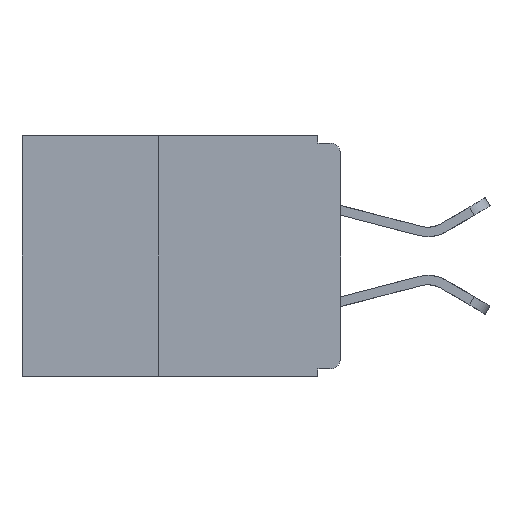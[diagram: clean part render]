
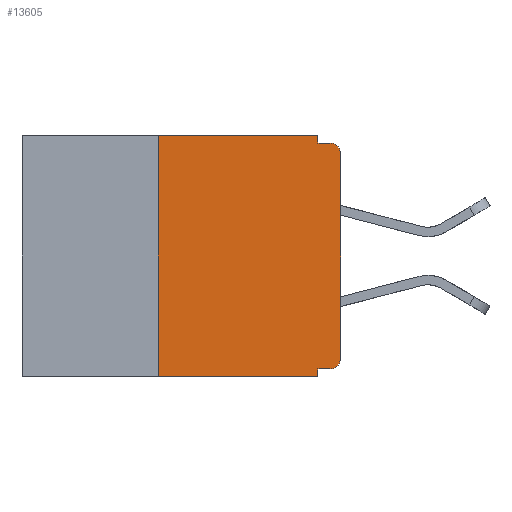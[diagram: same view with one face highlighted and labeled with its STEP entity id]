
A CAD part, left-side view. The second image highlights one B-rep face of the part: STEP entity #13605.
In plain terms, the highlighted planar face has unit normal (-1, 0, 0).
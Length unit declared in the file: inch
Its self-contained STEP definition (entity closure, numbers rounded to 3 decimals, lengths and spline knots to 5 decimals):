
#101 = EDGE_CURVE ( 'NONE', #22698, #2050, #8206, .T. ) ;
#167 = VECTOR ( 'NONE', #7514, 39.37008 ) ;
#479 = VERTEX_POINT ( 'NONE', #2441 ) ;
#530 = CARTESIAN_POINT ( 'NONE',  ( 0., 0., 0. ) ) ;
#1321 = CARTESIAN_POINT ( 'NONE',  ( 0., 0., -0.32 ) ) ;
#1730 = DIRECTION ( 'NONE',  ( 0., 0., -1. ) ) ;
#1799 = CARTESIAN_POINT ( 'NONE',  ( 0., 0.015, -0.025 ) ) ;
#2050 = VERTEX_POINT ( 'NONE', #16902 ) ;
#2095 = AXIS2_PLACEMENT_3D ( 'NONE', #2664, #7198, #19020 ) ;
#2288 = CARTESIAN_POINT ( 'NONE',  ( 0., 0.031, -0.32 ) ) ;
#2322 = LINE ( 'NONE', #14451, #21043 ) ;
#2324 = CARTESIAN_POINT ( 'NONE',  ( 0., 0.031, 0. ) ) ;
#2441 = CARTESIAN_POINT ( 'NONE',  ( 0., 0.015, -0.01 ) ) ;
#2648 = VERTEX_POINT ( 'NONE', #6542 ) ;
#2664 = CARTESIAN_POINT ( 'NONE',  ( 0., 0.015, -0.305 ) ) ;
#3255 = CARTESIAN_POINT ( 'NONE',  ( 0., 0.015, -0.32 ) ) ;
#3269 = DIRECTION ( 'NONE',  ( 0., 0., 1. ) ) ;
#3593 = ORIENTED_EDGE ( 'NONE', *, *, #8871, .F. ) ;
#3656 = DIRECTION ( 'NONE',  ( 0., 0., -1. ) ) ;
#3902 = EDGE_CURVE ( 'NONE', #22698, #8123, #21033, .T. ) ;
#4075 = VERTEX_POINT ( 'NONE', #5519 ) ;
#4183 = ORIENTED_EDGE ( 'NONE', *, *, #18935, .F. ) ;
#4959 = DIRECTION ( 'NONE',  ( 0., -1., 0. ) ) ;
#5228 = LINE ( 'NONE', #10748, #9482 ) ;
#5302 = LINE ( 'NONE', #22932, #19164 ) ;
#5373 = EDGE_CURVE ( 'NONE', #8123, #13644, #2322, .T. ) ;
#5519 = CARTESIAN_POINT ( 'NONE',  ( 0., 0.031, -0.01 ) ) ;
#5787 = EDGE_CURVE ( 'NONE', #16566, #9627, #17944, .T. ) ;
#6329 = EDGE_CURVE ( 'NONE', #2050, #7397, #15070, .T. ) ;
#6542 = CARTESIAN_POINT ( 'NONE',  ( 0., 0.031, 0. ) ) ;
#6786 = DIRECTION ( 'NONE',  ( 0., 1., 0. ) ) ;
#7198 = DIRECTION ( 'NONE',  ( -1., 0., 0. ) ) ;
#7209 = VECTOR ( 'NONE', #6786, 39.37008 ) ;
#7397 = VERTEX_POINT ( 'NONE', #16318 ) ;
#7514 = DIRECTION ( 'NONE',  ( 0., -1., 0. ) ) ;
#7894 = DIRECTION ( 'NONE',  ( 0., 0., 1. ) ) ;
#8123 = VERTEX_POINT ( 'NONE', #2288 ) ;
#8206 = CIRCLE ( 'NONE', #2095, 0.015 ) ;
#8225 = DIRECTION ( 'NONE',  ( 0., 0., -1. ) ) ;
#8871 = EDGE_CURVE ( 'NONE', #4075, #479, #18907, .T. ) ;
#9482 = VECTOR ( 'NONE', #12556, 39.37008 ) ;
#9627 = VERTEX_POINT ( 'NONE', #9699 ) ;
#9699 = CARTESIAN_POINT ( 'NONE',  ( 0., 0.25, 0. ) ) ;
#10141 = CARTESIAN_POINT ( 'NONE',  ( 0., 0.031, -0.33 ) ) ;
#10281 = VECTOR ( 'NONE', #7894, 39.37008 ) ;
#10460 = ORIENTED_EDGE ( 'NONE', *, *, #3902, .F. ) ;
#10507 = AXIS2_PLACEMENT_3D ( 'NONE', #1799, #14515, #3656 ) ;
#10579 = CARTESIAN_POINT ( 'NONE',  ( 0., 0.25, -0.33 ) ) ;
#10717 = AXIS2_PLACEMENT_3D ( 'NONE', #15425, #19064, #8225 ) ;
#10748 = CARTESIAN_POINT ( 'NONE',  ( 0., 0.437, -0.33 ) ) ;
#11400 = EDGE_LOOP ( 'NONE', ( #13207, #20298, #3593, #4183, #23113, #11551, #11854, #22020, #10460, #12442 ) ) ;
#11551 = ORIENTED_EDGE ( 'NONE', *, *, #5787, .F. ) ;
#11854 = ORIENTED_EDGE ( 'NONE', *, *, #22129, .T. ) ;
#12442 = ORIENTED_EDGE ( 'NONE', *, *, #101, .T. ) ;
#12551 = VECTOR ( 'NONE', #3269, 39.37008 ) ;
#12556 = DIRECTION ( 'NONE',  ( 0., -1., 0. ) ) ;
#12566 = EDGE_CURVE ( 'NONE', #9627, #2648, #5302, .T. ) ;
#13207 = ORIENTED_EDGE ( 'NONE', *, *, #6329, .T. ) ;
#13605 = ADVANCED_FACE ( 'NONE', ( #21943 ), #22583, .F. ) ;
#13644 = VERTEX_POINT ( 'NONE', #10141 ) ;
#14451 = CARTESIAN_POINT ( 'NONE',  ( 0., 0.031, -0.33 ) ) ;
#14515 = DIRECTION ( 'NONE',  ( -1., 0., 0. ) ) ;
#15070 = LINE ( 'NONE', #530, #10281 ) ;
#15425 = CARTESIAN_POINT ( 'NONE',  ( 0., 0.437, 0. ) ) ;
#16077 = CARTESIAN_POINT ( 'NONE',  ( 0., 0.25, -0.33 ) ) ;
#16318 = CARTESIAN_POINT ( 'NONE',  ( 0., 0., -0.025 ) ) ;
#16566 = VERTEX_POINT ( 'NONE', #16077 ) ;
#16868 = DIRECTION ( 'NONE',  ( 0., 0., -1. ) ) ;
#16902 = CARTESIAN_POINT ( 'NONE',  ( 0., 0., -0.305 ) ) ;
#16950 = LINE ( 'NONE', #2324, #22288 ) ;
#17180 = CIRCLE ( 'NONE', #10507, 0.015 ) ;
#17944 = LINE ( 'NONE', #10579, #12551 ) ;
#18907 = LINE ( 'NONE', #21954, #167 ) ;
#18935 = EDGE_CURVE ( 'NONE', #2648, #4075, #16950, .T. ) ;
#19020 = DIRECTION ( 'NONE',  ( 0., 0., -1. ) ) ;
#19064 = DIRECTION ( 'NONE',  ( 1., 0., 0. ) ) ;
#19164 = VECTOR ( 'NONE', #4959, 39.37008 ) ;
#20012 = EDGE_CURVE ( 'NONE', #7397, #479, #17180, .T. ) ;
#20298 = ORIENTED_EDGE ( 'NONE', *, *, #20012, .T. ) ;
#21033 = LINE ( 'NONE', #1321, #7209 ) ;
#21043 = VECTOR ( 'NONE', #1730, 39.37008 ) ;
#21943 = FACE_OUTER_BOUND ( 'NONE', #11400, .T. ) ;
#21954 = CARTESIAN_POINT ( 'NONE',  ( 0., 0., -0.01 ) ) ;
#22020 = ORIENTED_EDGE ( 'NONE', *, *, #5373, .F. ) ;
#22129 = EDGE_CURVE ( 'NONE', #16566, #13644, #5228, .T. ) ;
#22288 = VECTOR ( 'NONE', #16868, 39.37008 ) ;
#22583 = PLANE ( 'NONE',  #10717 ) ;
#22698 = VERTEX_POINT ( 'NONE', #3255 ) ;
#22932 = CARTESIAN_POINT ( 'NONE',  ( 0., 0.437, 0. ) ) ;
#23113 = ORIENTED_EDGE ( 'NONE', *, *, #12566, .F. ) ;
